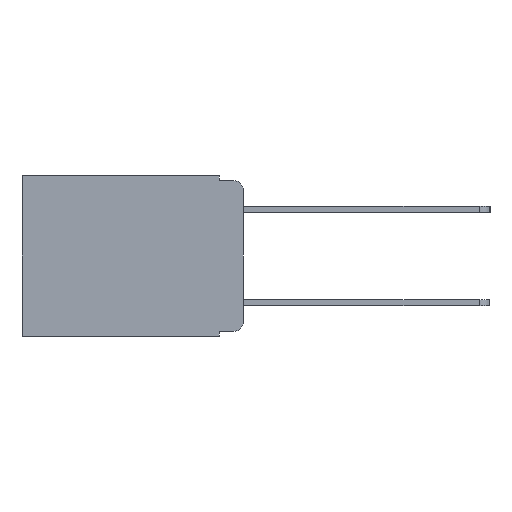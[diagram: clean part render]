
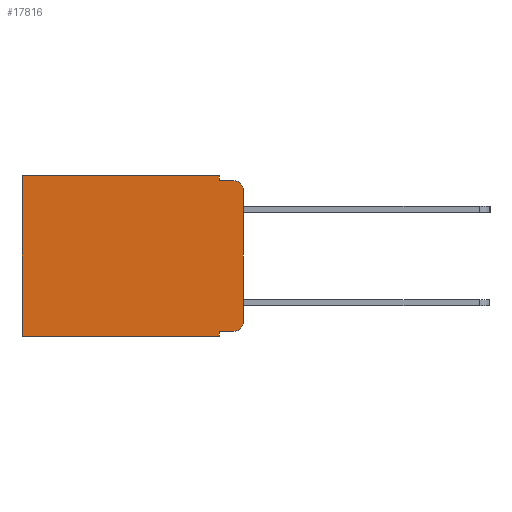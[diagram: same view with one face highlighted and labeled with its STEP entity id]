
A CAD part, left-side view. The second image highlights one B-rep face of the part: STEP entity #17816.
In plain terms, the highlighted planar face has unit normal (-1, 0, 0).
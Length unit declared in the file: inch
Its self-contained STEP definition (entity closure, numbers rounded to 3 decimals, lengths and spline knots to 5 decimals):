
#14 = CARTESIAN_POINT ( 'NONE',  ( 0.298, 0.473, 0. ) ) ;
#54 = CARTESIAN_POINT ( 'NONE',  ( 0.298, 0.051, -0.01 ) ) ;
#133 = LINE ( 'NONE', #15902, #12125 ) ;
#718 = DIRECTION ( 'NONE',  ( 0., 0., -1. ) ) ;
#797 = EDGE_CURVE ( 'NONE', #7875, #15357, #17910, .T. ) ;
#1088 = VECTOR ( 'NONE', #12471, 39.37008 ) ;
#1208 = VECTOR ( 'NONE', #1211, 39.37008 ) ;
#1211 = DIRECTION ( 'NONE',  ( 0., 1., 0. ) ) ;
#1596 = LINE ( 'NONE', #5373, #1088 ) ;
#2078 = VERTEX_POINT ( 'NONE', #17985 ) ;
#2554 = VERTEX_POINT ( 'NONE', #9793 ) ;
#2935 = VECTOR ( 'NONE', #718, 39.37008 ) ;
#3329 = EDGE_LOOP ( 'NONE', ( #11248, #12046, #12126, #11972, #13206, #13086, #12919, #12709, #12648, #12616 ) ) ;
#3386 = VECTOR ( 'NONE', #9453, 39.37008 ) ;
#3704 = AXIS2_PLACEMENT_3D ( 'NONE', #4852, #15503, #6403 ) ;
#4275 = EDGE_CURVE ( 'NONE', #5845, #9761, #1596, .T. ) ;
#4307 = DIRECTION ( 'NONE',  ( 1., 0., 0. ) ) ;
#4852 = CARTESIAN_POINT ( 'NONE',  ( 0.298, 0.02, -0.03 ) ) ;
#4877 = DIRECTION ( 'NONE',  ( 0., -1., 0. ) ) ;
#5286 = AXIS2_PLACEMENT_3D ( 'NONE', #17849, #17835, #17274 ) ;
#5304 = CARTESIAN_POINT ( 'NONE',  ( 0.298, 0., -0.313 ) ) ;
#5310 = EDGE_CURVE ( 'NONE', #9905, #9761, #9895, .T. ) ;
#5373 = CARTESIAN_POINT ( 'NONE',  ( 0.298, 0., 0. ) ) ;
#5590 = LINE ( 'NONE', #13335, #13754 ) ;
#5845 = VERTEX_POINT ( 'NONE', #18865 ) ;
#5920 = VECTOR ( 'NONE', #4877, 39.37008 ) ;
#6348 = EDGE_CURVE ( 'NONE', #2078, #12326, #7233, .T. ) ;
#6403 = DIRECTION ( 'NONE',  ( 0., 0., -1. ) ) ;
#6405 = LINE ( 'NONE', #54, #5920 ) ;
#6691 = CARTESIAN_POINT ( 'NONE',  ( 0.298, 0., -0.343 ) ) ;
#7233 = LINE ( 'NONE', #9900, #14844 ) ;
#7560 = LINE ( 'NONE', #11629, #2935 ) ;
#7875 = VERTEX_POINT ( 'NONE', #11994 ) ;
#8767 = DIRECTION ( 'NONE',  ( 0., -1., 0. ) ) ;
#9453 = DIRECTION ( 'NONE',  ( 0., 0., -1. ) ) ;
#9761 = VERTEX_POINT ( 'NONE', #5304 ) ;
#9793 = CARTESIAN_POINT ( 'NONE',  ( 0.298, 0.473, 0. ) ) ;
#9895 = CIRCLE ( 'NONE', #5286, 0.02 ) ;
#9900 = CARTESIAN_POINT ( 'NONE',  ( 0.298, 0.051, 0. ) ) ;
#9905 = VERTEX_POINT ( 'NONE', #11714 ) ;
#10348 = EDGE_CURVE ( 'NONE', #2078, #2554, #133, .T. ) ;
#10422 = EDGE_CURVE ( 'NONE', #18760, #7875, #7560, .T. ) ;
#10467 = CARTESIAN_POINT ( 'NONE',  ( 0.298, 0., 0. ) ) ;
#10503 = EDGE_CURVE ( 'NONE', #18760, #9905, #5590, .T. ) ;
#11248 = ORIENTED_EDGE ( 'NONE', *, *, #4275, .F. ) ;
#11629 = CARTESIAN_POINT ( 'NONE',  ( 0.298, 0.051, 0. ) ) ;
#11714 = CARTESIAN_POINT ( 'NONE',  ( 0.298, 0.02, -0.333 ) ) ;
#11863 = CARTESIAN_POINT ( 'NONE',  ( 0.298, 0.051, -0.01 ) ) ;
#11972 = ORIENTED_EDGE ( 'NONE', *, *, #6348, .F. ) ;
#11994 = CARTESIAN_POINT ( 'NONE',  ( 0.298, 0.051, -0.343 ) ) ;
#12046 = ORIENTED_EDGE ( 'NONE', *, *, #13905, .T. ) ;
#12125 = VECTOR ( 'NONE', #14375, 39.37008 ) ;
#12126 = ORIENTED_EDGE ( 'NONE', *, *, #14907, .F. ) ;
#12326 = VERTEX_POINT ( 'NONE', #11863 ) ;
#12471 = DIRECTION ( 'NONE',  ( 0., 0., -1. ) ) ;
#12482 = CIRCLE ( 'NONE', #3704, 0.02 ) ;
#12616 = ORIENTED_EDGE ( 'NONE', *, *, #5310, .T. ) ;
#12648 = ORIENTED_EDGE ( 'NONE', *, *, #10503, .T. ) ;
#12709 = ORIENTED_EDGE ( 'NONE', *, *, #10422, .F. ) ;
#12919 = ORIENTED_EDGE ( 'NONE', *, *, #797, .F. ) ;
#12949 = VERTEX_POINT ( 'NONE', #19038 ) ;
#13086 = ORIENTED_EDGE ( 'NONE', *, *, #19121, .T. ) ;
#13206 = ORIENTED_EDGE ( 'NONE', *, *, #10348, .T. ) ;
#13335 = CARTESIAN_POINT ( 'NONE',  ( 0.298, 0.051, -0.333 ) ) ;
#13754 = VECTOR ( 'NONE', #8767, 39.37008 ) ;
#13782 = CARTESIAN_POINT ( 'NONE',  ( 0.298, 0.473, -0.343 ) ) ;
#13905 = EDGE_CURVE ( 'NONE', #5845, #12949, #12482, .T. ) ;
#14375 = DIRECTION ( 'NONE',  ( 0., 1., 0. ) ) ;
#14844 = VECTOR ( 'NONE', #18787, 39.37008 ) ;
#14907 = EDGE_CURVE ( 'NONE', #12326, #12949, #6405, .T. ) ;
#14982 = FACE_OUTER_BOUND ( 'NONE', #3329, .T. ) ;
#15004 = DIRECTION ( 'NONE',  ( 0., 0., -1. ) ) ;
#15357 = VERTEX_POINT ( 'NONE', #13782 ) ;
#15503 = DIRECTION ( 'NONE',  ( -1., 0., 0. ) ) ;
#15649 = CARTESIAN_POINT ( 'NONE',  ( 0.298, 0.051, -0.333 ) ) ;
#15902 = CARTESIAN_POINT ( 'NONE',  ( 0.298, 0., 0. ) ) ;
#16402 = PLANE ( 'NONE',  #17110 ) ;
#17110 = AXIS2_PLACEMENT_3D ( 'NONE', #10467, #4307, #15004 ) ;
#17274 = DIRECTION ( 'NONE',  ( 0., 0., -1. ) ) ;
#17816 = ADVANCED_FACE ( 'NONE', ( #14982 ), #16402, .F. ) ;
#17835 = DIRECTION ( 'NONE',  ( -1., 0., 0. ) ) ;
#17849 = CARTESIAN_POINT ( 'NONE',  ( 0.298, 0.02, -0.313 ) ) ;
#17910 = LINE ( 'NONE', #6691, #1208 ) ;
#17985 = CARTESIAN_POINT ( 'NONE',  ( 0.298, 0.051, 0. ) ) ;
#18760 = VERTEX_POINT ( 'NONE', #15649 ) ;
#18787 = DIRECTION ( 'NONE',  ( 0., 0., -1. ) ) ;
#18865 = CARTESIAN_POINT ( 'NONE',  ( 0.298, 0., -0.03 ) ) ;
#18986 = LINE ( 'NONE', #14, #3386 ) ;
#19038 = CARTESIAN_POINT ( 'NONE',  ( 0.298, 0.02, -0.01 ) ) ;
#19121 = EDGE_CURVE ( 'NONE', #2554, #15357, #18986, .T. ) ;
